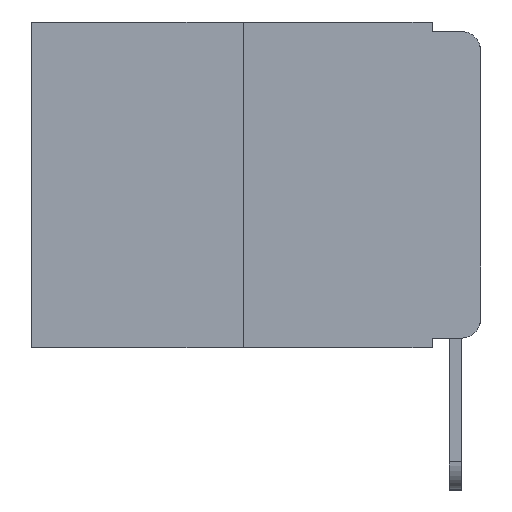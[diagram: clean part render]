
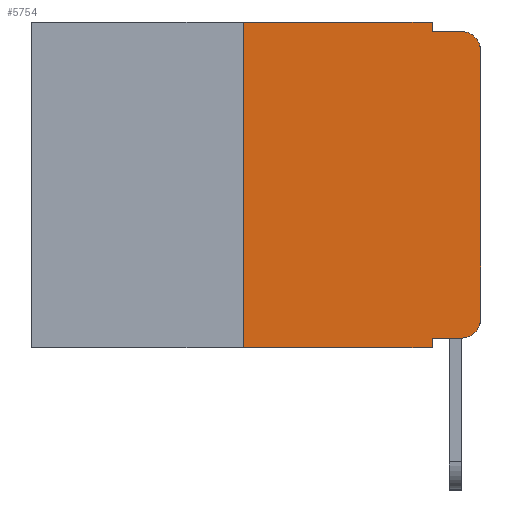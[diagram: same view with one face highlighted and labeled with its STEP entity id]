
A CAD part, left-side view. The second image highlights one B-rep face of the part: STEP entity #5754.
In plain terms, the highlighted planar face has unit normal (-1, 0, 0).
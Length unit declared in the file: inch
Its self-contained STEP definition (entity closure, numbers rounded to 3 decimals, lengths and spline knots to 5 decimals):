
#342 = VERTEX_POINT ( 'NONE', #10857 ) ;
#1058 = DIRECTION ( 'NONE',  ( 0., -1., 0. ) ) ;
#1106 = CARTESIAN_POINT ( 'NONE',  ( 0., 0.02, -0.333 ) ) ;
#1146 = CARTESIAN_POINT ( 'NONE',  ( 0., 0.25, 0. ) ) ;
#1148 = ORIENTED_EDGE ( 'NONE', *, *, #2968, .F. ) ;
#1197 = DIRECTION ( 'NONE',  ( -1., 0., 0. ) ) ;
#1370 = VECTOR ( 'NONE', #11202, 39.37008 ) ;
#1576 = VERTEX_POINT ( 'NONE', #12051 ) ;
#2039 = VECTOR ( 'NONE', #17736, 39.37008 ) ;
#2072 = LINE ( 'NONE', #5149, #5139 ) ;
#2240 = CARTESIAN_POINT ( 'NONE',  ( 0., 0.051, 0. ) ) ;
#2256 = PLANE ( 'NONE',  #5240 ) ;
#2358 = ORIENTED_EDGE ( 'NONE', *, *, #12655, .T. ) ;
#2767 = EDGE_CURVE ( 'NONE', #18616, #12664, #12749, .T. ) ;
#2858 = CARTESIAN_POINT ( 'NONE',  ( 0., 0.02, -0.313 ) ) ;
#2968 = EDGE_CURVE ( 'NONE', #3034, #18616, #2072, .T. ) ;
#3034 = VERTEX_POINT ( 'NONE', #2240 ) ;
#3412 = ORIENTED_EDGE ( 'NONE', *, *, #13957, .T. ) ;
#3586 = CARTESIAN_POINT ( 'NONE',  ( 0., 0.02, -0.01 ) ) ;
#4650 = VERTEX_POINT ( 'NONE', #10015 ) ;
#5139 = VECTOR ( 'NONE', #6691, 39.37008 ) ;
#5149 = CARTESIAN_POINT ( 'NONE',  ( 0., 0.051, 0. ) ) ;
#5240 = AXIS2_PLACEMENT_3D ( 'NONE', #14304, #9876, #11268 ) ;
#5754 = ADVANCED_FACE ( 'NONE', ( #11781 ), #2256, .F. ) ;
#5913 = CARTESIAN_POINT ( 'NONE',  ( 0., 0.051, -0.01 ) ) ;
#6014 = ORIENTED_EDGE ( 'NONE', *, *, #10667, .F. ) ;
#6280 = CARTESIAN_POINT ( 'NONE',  ( 0., 0., -0.03 ) ) ;
#6462 = DIRECTION ( 'NONE',  ( 0., 0., -1. ) ) ;
#6586 = CARTESIAN_POINT ( 'NONE',  ( 0., 0.25, 0. ) ) ;
#6691 = DIRECTION ( 'NONE',  ( 0., 0., -1. ) ) ;
#6925 = DIRECTION ( 'NONE',  ( 0., -1., 0. ) ) ;
#8066 = VECTOR ( 'NONE', #16463, 39.37008 ) ;
#8072 = DIRECTION ( 'NONE',  ( -1., 0., 0. ) ) ;
#8126 = EDGE_CURVE ( 'NONE', #1576, #342, #16310, .T. ) ;
#8210 = CARTESIAN_POINT ( 'NONE',  ( 0., 0., 0. ) ) ;
#8919 = VERTEX_POINT ( 'NONE', #6586 ) ;
#9340 = EDGE_CURVE ( 'NONE', #14560, #12664, #10038, .T. ) ;
#9770 = ORIENTED_EDGE ( 'NONE', *, *, #8126, .T. ) ;
#9876 = DIRECTION ( 'NONE',  ( 1., 0., 0. ) ) ;
#9964 = CARTESIAN_POINT ( 'NONE',  ( 0., 0.051, -0.333 ) ) ;
#10015 = CARTESIAN_POINT ( 'NONE',  ( 0., 0.051, -0.333 ) ) ;
#10038 = CIRCLE ( 'NONE', #10792, 0.02 ) ;
#10147 = LINE ( 'NONE', #8210, #1370 ) ;
#10554 = LINE ( 'NONE', #9964, #18249 ) ;
#10667 = EDGE_CURVE ( 'NONE', #4650, #342, #15727, .T. ) ;
#10792 = AXIS2_PLACEMENT_3D ( 'NONE', #15544, #8072, #18657 ) ;
#10819 = AXIS2_PLACEMENT_3D ( 'NONE', #2858, #1197, #19450 ) ;
#10857 = CARTESIAN_POINT ( 'NONE',  ( 0., 0.051, -0.343 ) ) ;
#11202 = DIRECTION ( 'NONE',  ( 0., 0., 1. ) ) ;
#11268 = DIRECTION ( 'NONE',  ( 0., 0., -1. ) ) ;
#11312 = ORIENTED_EDGE ( 'NONE', *, *, #12869, .T. ) ;
#11509 = EDGE_LOOP ( 'NONE', ( #2358, #13254, #12161, #1148, #14606, #18852, #9770, #6014, #3412, #11312 ) ) ;
#11657 = CARTESIAN_POINT ( 'NONE',  ( 0., 0., -0.313 ) ) ;
#11781 = FACE_OUTER_BOUND ( 'NONE', #11509, .T. ) ;
#12051 = CARTESIAN_POINT ( 'NONE',  ( 0., 0.25, -0.343 ) ) ;
#12137 = LINE ( 'NONE', #1146, #8066 ) ;
#12161 = ORIENTED_EDGE ( 'NONE', *, *, #2767, .F. ) ;
#12375 = CARTESIAN_POINT ( 'NONE',  ( 0., 0.051, -0.01 ) ) ;
#12489 = CARTESIAN_POINT ( 'NONE',  ( 0., 0.051, 0. ) ) ;
#12655 = EDGE_CURVE ( 'NONE', #16225, #14560, #10147, .T. ) ;
#12664 = VERTEX_POINT ( 'NONE', #3586 ) ;
#12749 = LINE ( 'NONE', #5913, #19736 ) ;
#12869 = EDGE_CURVE ( 'NONE', #16302, #16225, #19734, .T. ) ;
#13254 = ORIENTED_EDGE ( 'NONE', *, *, #9340, .T. ) ;
#13957 = EDGE_CURVE ( 'NONE', #4650, #16302, #10554, .T. ) ;
#14064 = VECTOR ( 'NONE', #6462, 39.37008 ) ;
#14304 = CARTESIAN_POINT ( 'NONE',  ( 0., 0.473, 0. ) ) ;
#14560 = VERTEX_POINT ( 'NONE', #6280 ) ;
#14606 = ORIENTED_EDGE ( 'NONE', *, *, #19453, .F. ) ;
#15544 = CARTESIAN_POINT ( 'NONE',  ( 0., 0.02, -0.03 ) ) ;
#15727 = LINE ( 'NONE', #12489, #14064 ) ;
#16225 = VERTEX_POINT ( 'NONE', #11657 ) ;
#16302 = VERTEX_POINT ( 'NONE', #1106 ) ;
#16310 = LINE ( 'NONE', #17665, #18015 ) ;
#16463 = DIRECTION ( 'NONE',  ( 0., 0., 1. ) ) ;
#16977 = EDGE_CURVE ( 'NONE', #1576, #8919, #12137, .T. ) ;
#17548 = LINE ( 'NONE', #17669, #2039 ) ;
#17665 = CARTESIAN_POINT ( 'NONE',  ( 0., 0.473, -0.343 ) ) ;
#17669 = CARTESIAN_POINT ( 'NONE',  ( 0., 0.473, 0. ) ) ;
#17736 = DIRECTION ( 'NONE',  ( 0., -1., 0. ) ) ;
#18015 = VECTOR ( 'NONE', #1058, 39.37008 ) ;
#18249 = VECTOR ( 'NONE', #6925, 39.37008 ) ;
#18616 = VERTEX_POINT ( 'NONE', #12375 ) ;
#18657 = DIRECTION ( 'NONE',  ( 0., 0., -1. ) ) ;
#18852 = ORIENTED_EDGE ( 'NONE', *, *, #16977, .F. ) ;
#19450 = DIRECTION ( 'NONE',  ( 0., 0., -1. ) ) ;
#19453 = EDGE_CURVE ( 'NONE', #8919, #3034, #17548, .T. ) ;
#19724 = DIRECTION ( 'NONE',  ( 0., -1., 0. ) ) ;
#19734 = CIRCLE ( 'NONE', #10819, 0.02 ) ;
#19736 = VECTOR ( 'NONE', #19724, 39.37008 ) ;
